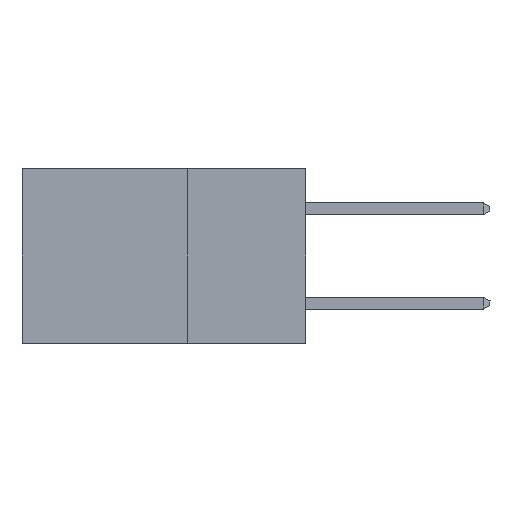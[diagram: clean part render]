
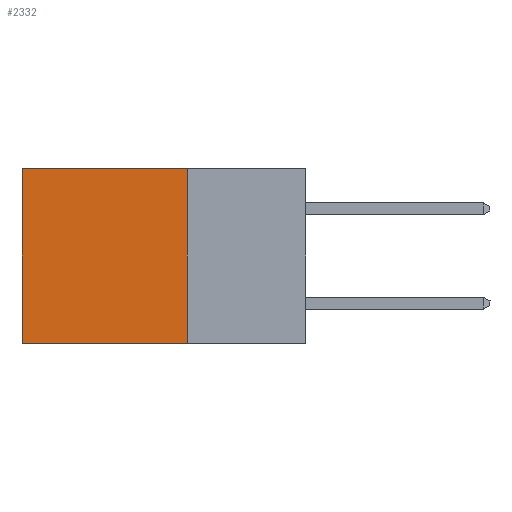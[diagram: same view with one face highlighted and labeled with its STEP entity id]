
A CAD part, left-side view. The second image highlights one B-rep face of the part: STEP entity #2332.
In plain terms, the highlighted planar face has unit normal (-1, 0, 0).
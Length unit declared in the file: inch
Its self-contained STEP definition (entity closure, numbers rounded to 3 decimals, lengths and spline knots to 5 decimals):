
#8 = VERTEX_POINT ( 'NONE', #12895 ) ;
#369 = AXIS2_PLACEMENT_3D ( 'NONE', #1512, #2713, #8054 ) ;
#646 = DIRECTION ( 'NONE',  ( 0., 1., 0. ) ) ;
#664 = CARTESIAN_POINT ( 'NONE',  ( 0.298, 0.25, 0. ) ) ;
#824 = ORIENTED_EDGE ( 'NONE', *, *, #1918, .F. ) ;
#1482 = VERTEX_POINT ( 'NONE', #8541 ) ;
#1512 = CARTESIAN_POINT ( 'NONE',  ( 0.298, 0.25, 0. ) ) ;
#1675 = CARTESIAN_POINT ( 'NONE',  ( 0.298, 0.25, 0. ) ) ;
#1693 = DIRECTION ( 'NONE',  ( 0., 0., -1. ) ) ;
#1918 = EDGE_CURVE ( 'NONE', #8, #1482, #6745, .T. ) ;
#2332 = ADVANCED_FACE ( 'NONE', ( #12743 ), #10982, .F. ) ;
#2713 = DIRECTION ( 'NONE',  ( 1., 0., 0. ) ) ;
#3073 = ORIENTED_EDGE ( 'NONE', *, *, #12001, .F. ) ;
#5047 = CARTESIAN_POINT ( 'NONE',  ( 0.298, 0.25, -0.37 ) ) ;
#5085 = EDGE_LOOP ( 'NONE', ( #5375, #824, #3073, #10007 ) ) ;
#5375 = ORIENTED_EDGE ( 'NONE', *, *, #5526, .T. ) ;
#5526 = EDGE_CURVE ( 'NONE', #7796, #1482, #13451, .T. ) ;
#5984 = CARTESIAN_POINT ( 'NONE',  ( 0.298, 0.25, 0. ) ) ;
#6690 = LINE ( 'NONE', #664, #7699 ) ;
#6745 = LINE ( 'NONE', #5047, #9575 ) ;
#6780 = VERTEX_POINT ( 'NONE', #1675 ) ;
#6814 = LINE ( 'NONE', #5984, #10651 ) ;
#6881 = DIRECTION ( 'NONE',  ( 0., 0., -1. ) ) ;
#7680 = CARTESIAN_POINT ( 'NONE',  ( 0.298, 0.6, 0. ) ) ;
#7699 = VECTOR ( 'NONE', #6881, 39.37008 ) ;
#7796 = VERTEX_POINT ( 'NONE', #7680 ) ;
#8054 = DIRECTION ( 'NONE',  ( 0., 0., -1. ) ) ;
#8288 = VECTOR ( 'NONE', #1693, 39.37008 ) ;
#8541 = CARTESIAN_POINT ( 'NONE',  ( 0.298, 0.6, -0.37 ) ) ;
#8775 = EDGE_CURVE ( 'NONE', #6780, #7796, #6814, .T. ) ;
#9575 = VECTOR ( 'NONE', #12503, 39.37008 ) ;
#10007 = ORIENTED_EDGE ( 'NONE', *, *, #8775, .T. ) ;
#10651 = VECTOR ( 'NONE', #646, 39.37008 ) ;
#10982 = PLANE ( 'NONE',  #369 ) ;
#12001 = EDGE_CURVE ( 'NONE', #6780, #8, #6690, .T. ) ;
#12199 = CARTESIAN_POINT ( 'NONE',  ( 0.298, 0.6, 0. ) ) ;
#12503 = DIRECTION ( 'NONE',  ( 0., 1., 0. ) ) ;
#12743 = FACE_OUTER_BOUND ( 'NONE', #5085, .T. ) ;
#12895 = CARTESIAN_POINT ( 'NONE',  ( 0.298, 0.25, -0.37 ) ) ;
#13451 = LINE ( 'NONE', #12199, #8288 ) ;
